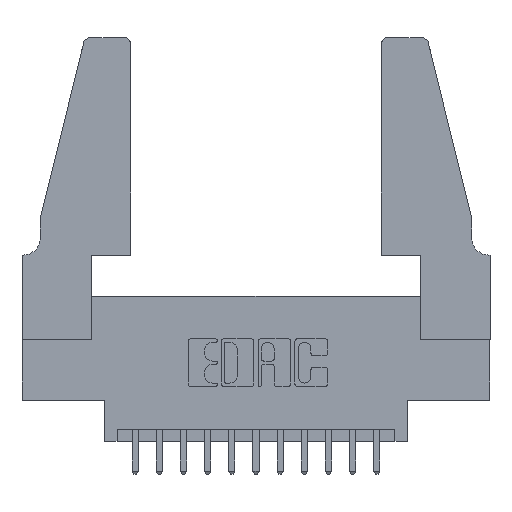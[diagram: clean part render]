
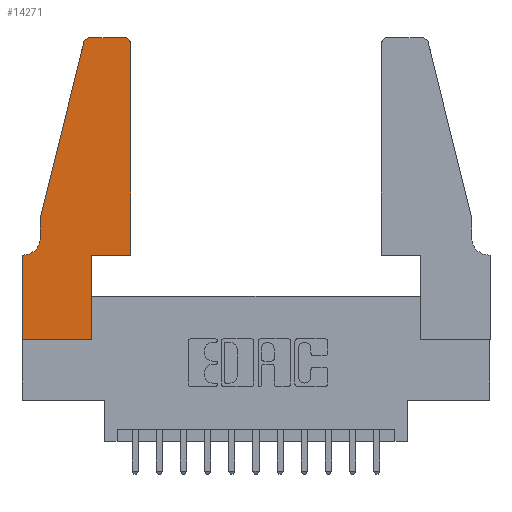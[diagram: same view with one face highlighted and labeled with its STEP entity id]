
A CAD part, top view. The second image highlights one B-rep face of the part: STEP entity #14271.
In plain terms, the highlighted planar face has unit normal (0, 0, 1).
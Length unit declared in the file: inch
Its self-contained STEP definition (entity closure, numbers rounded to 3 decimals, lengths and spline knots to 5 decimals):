
#88 = DIRECTION ( 'NONE',  ( 0., 0., 1. ) ) ;
#192 = LINE ( 'NONE', #12729, #948 ) ;
#575 = DIRECTION ( 'NONE',  ( 0., 1., 0. ) ) ;
#581 = CARTESIAN_POINT ( 'NONE',  ( 0., 0., 0.37 ) ) ;
#671 = ORIENTED_EDGE ( 'NONE', *, *, #3834, .T. ) ;
#924 = CARTESIAN_POINT ( 'NONE',  ( 0.0755, 0.35, 0.37 ) ) ;
#948 = VECTOR ( 'NONE', #949, 39.37008 ) ;
#949 = DIRECTION ( 'NONE',  ( 0., -1., 0. ) ) ;
#1162 = LINE ( 'NONE', #11492, #1705 ) ;
#1186 = EDGE_CURVE ( 'NONE', #10573, #3371, #3174, .T. ) ;
#1257 = CARTESIAN_POINT ( 'NONE',  ( 0.284, 1.22, 0.37 ) ) ;
#1312 = DIRECTION ( 'NONE',  ( -0.239, -0.971, 0. ) ) ;
#1385 = CARTESIAN_POINT ( 'NONE',  ( 0.0755, 0.5, 0.37 ) ) ;
#1664 = CARTESIAN_POINT ( 'NONE',  ( 0.284, 1.25, 0.37 ) ) ;
#1705 = VECTOR ( 'NONE', #3178, 39.37008 ) ;
#2236 = DIRECTION ( 'NONE',  ( 1., 0., 0. ) ) ;
#2277 = CARTESIAN_POINT ( 'NONE',  ( 0.2865, 0.35, 0.37 ) ) ;
#2279 = CARTESIAN_POINT ( 'NONE',  ( 0.0055, 0.35, 0.37 ) ) ;
#2411 = EDGE_CURVE ( 'NONE', #12925, #8163, #192, .T. ) ;
#2416 = VECTOR ( 'NONE', #3584, 39.37008 ) ;
#2598 = CARTESIAN_POINT ( 'NONE',  ( 0.2865, 0., 0.37 ) ) ;
#2884 = CARTESIAN_POINT ( 'NONE',  ( 0.4505, 0.35, 0.37 ) ) ;
#2936 = DIRECTION ( 'NONE',  ( 0., 0., 1. ) ) ;
#2974 = LINE ( 'NONE', #924, #10500 ) ;
#3120 = LINE ( 'NONE', #12266, #7152 ) ;
#3174 = LINE ( 'NONE', #11731, #7960 ) ;
#3178 = DIRECTION ( 'NONE',  ( 0., -1., 0. ) ) ;
#3371 = VERTEX_POINT ( 'NONE', #2598 ) ;
#3584 = DIRECTION ( 'NONE',  ( 1., 0., 0. ) ) ;
#3618 = ORIENTED_EDGE ( 'NONE', *, *, #15112, .T. ) ;
#3650 = VERTEX_POINT ( 'NONE', #11408 ) ;
#3834 = EDGE_CURVE ( 'NONE', #3650, #9196, #10665, .T. ) ;
#3977 = VERTEX_POINT ( 'NONE', #12471 ) ;
#4043 = LINE ( 'NONE', #2884, #2416 ) ;
#4058 = LINE ( 'NONE', #9718, #5722 ) ;
#4734 = DIRECTION ( 'NONE',  ( 0., 0., 1. ) ) ;
#4767 = ORIENTED_EDGE ( 'NONE', *, *, #7226, .T. ) ;
#5014 = ORIENTED_EDGE ( 'NONE', *, *, #8729, .T. ) ;
#5121 = ORIENTED_EDGE ( 'NONE', *, *, #2411, .T. ) ;
#5150 = VECTOR ( 'NONE', #13228, 39.37008 ) ;
#5338 = CARTESIAN_POINT ( 'NONE',  ( 0.4205, 1.22, 0.37 ) ) ;
#5374 = EDGE_LOOP ( 'NONE', ( #671, #12366, #10784, #5121, #4767, #5014, #10642, #8195, #13845, #10178, #3618, #6887 ) ) ;
#5722 = VECTOR ( 'NONE', #1312, 39.37008 ) ;
#5810 = EDGE_CURVE ( 'NONE', #14382, #3650, #12967, .T. ) ;
#6141 = AXIS2_PLACEMENT_3D ( 'NONE', #11034, #10040, #14878 ) ;
#6171 = CIRCLE ( 'NONE', #6141, 0.07 ) ;
#6328 = CARTESIAN_POINT ( 'NONE',  ( 0.0755, 0.42, 0.37 ) ) ;
#6430 = AXIS2_PLACEMENT_3D ( 'NONE', #1257, #88, #6917 ) ;
#6494 = VERTEX_POINT ( 'NONE', #2279 ) ;
#6688 = CARTESIAN_POINT ( 'NONE',  ( 0.4505, 1.22, 0.37 ) ) ;
#6723 = DIRECTION ( 'NONE',  ( -1., 0., 0. ) ) ;
#6887 = ORIENTED_EDGE ( 'NONE', *, *, #5810, .T. ) ;
#6917 = DIRECTION ( 'NONE',  ( 1., 0., 0. ) ) ;
#7152 = VECTOR ( 'NONE', #575, 39.37008 ) ;
#7226 = EDGE_CURVE ( 'NONE', #8163, #6494, #6171, .T. ) ;
#7960 = VECTOR ( 'NONE', #2236, 39.37008 ) ;
#8013 = AXIS2_PLACEMENT_3D ( 'NONE', #5338, #2936, #13364 ) ;
#8149 = VERTEX_POINT ( 'NONE', #11605 ) ;
#8163 = VERTEX_POINT ( 'NONE', #6328 ) ;
#8195 = ORIENTED_EDGE ( 'NONE', *, *, #1186, .T. ) ;
#8222 = EDGE_CURVE ( 'NONE', #8668, #10573, #1162, .T. ) ;
#8668 = VERTEX_POINT ( 'NONE', #9050 ) ;
#8724 = CARTESIAN_POINT ( 'NONE',  ( 0.2605, 1.25, 0.37 ) ) ;
#8729 = EDGE_CURVE ( 'NONE', #6494, #8668, #2974, .T. ) ;
#8747 = FACE_OUTER_BOUND ( 'NONE', #5374, .T. ) ;
#8976 = EDGE_CURVE ( 'NONE', #8149, #12925, #4058, .T. ) ;
#9050 = CARTESIAN_POINT ( 'NONE',  ( 0., 0.35, 0.37 ) ) ;
#9196 = VERTEX_POINT ( 'NONE', #1664 ) ;
#9273 = LINE ( 'NONE', #11637, #9459 ) ;
#9459 = VECTOR ( 'NONE', #13902, 39.37008 ) ;
#9718 = CARTESIAN_POINT ( 'NONE',  ( 0.0755, 0.5, 0.37 ) ) ;
#9869 = CIRCLE ( 'NONE', #6430, 0.03 ) ;
#10033 = AXIS2_PLACEMENT_3D ( 'NONE', #15058, #4734, #11684 ) ;
#10040 = DIRECTION ( 'NONE',  ( 0., 0., -1. ) ) ;
#10178 = ORIENTED_EDGE ( 'NONE', *, *, #11085, .T. ) ;
#10500 = VECTOR ( 'NONE', #6723, 39.37008 ) ;
#10573 = VERTEX_POINT ( 'NONE', #581 ) ;
#10600 = PLANE ( 'NONE',  #10033 ) ;
#10642 = ORIENTED_EDGE ( 'NONE', *, *, #8222, .T. ) ;
#10665 = LINE ( 'NONE', #8724, #5150 ) ;
#10784 = ORIENTED_EDGE ( 'NONE', *, *, #8976, .T. ) ;
#11034 = CARTESIAN_POINT ( 'NONE',  ( 0.0055, 0.42, 0.37 ) ) ;
#11085 = EDGE_CURVE ( 'NONE', #12309, #3977, #4043, .T. ) ;
#11408 = CARTESIAN_POINT ( 'NONE',  ( 0.4205, 1.25, 0.37 ) ) ;
#11492 = CARTESIAN_POINT ( 'NONE',  ( 0., 0., 0.37 ) ) ;
#11605 = CARTESIAN_POINT ( 'NONE',  ( 0.25487, 1.22718, 0.37 ) ) ;
#11637 = CARTESIAN_POINT ( 'NONE',  ( 0.4505, 0.35, 0.37 ) ) ;
#11684 = DIRECTION ( 'NONE',  ( 1., 0., 0. ) ) ;
#11731 = CARTESIAN_POINT ( 'NONE',  ( 0., 0., 0.37 ) ) ;
#12266 = CARTESIAN_POINT ( 'NONE',  ( 0.2865, 0.35, 0.37 ) ) ;
#12309 = VERTEX_POINT ( 'NONE', #2277 ) ;
#12366 = ORIENTED_EDGE ( 'NONE', *, *, #14230, .T. ) ;
#12469 = EDGE_CURVE ( 'NONE', #3371, #12309, #3120, .T. ) ;
#12471 = CARTESIAN_POINT ( 'NONE',  ( 0.4505, 0.35, 0.37 ) ) ;
#12729 = CARTESIAN_POINT ( 'NONE',  ( 0.0755, 0.5, 0.37 ) ) ;
#12925 = VERTEX_POINT ( 'NONE', #1385 ) ;
#12967 = CIRCLE ( 'NONE', #8013, 0.03 ) ;
#13228 = DIRECTION ( 'NONE',  ( -1., 0., 0. ) ) ;
#13364 = DIRECTION ( 'NONE',  ( 1., 0., 0. ) ) ;
#13845 = ORIENTED_EDGE ( 'NONE', *, *, #12469, .T. ) ;
#13902 = DIRECTION ( 'NONE',  ( 0., 1., 0. ) ) ;
#14230 = EDGE_CURVE ( 'NONE', #9196, #8149, #9869, .T. ) ;
#14271 = ADVANCED_FACE ( 'NONE', ( #8747 ), #10600, .T. ) ;
#14382 = VERTEX_POINT ( 'NONE', #6688 ) ;
#14878 = DIRECTION ( 'NONE',  ( -1., 0., 0. ) ) ;
#15058 = CARTESIAN_POINT ( 'NONE',  ( 0., 0.35, 0.37 ) ) ;
#15112 = EDGE_CURVE ( 'NONE', #3977, #14382, #9273, .T. ) ;
